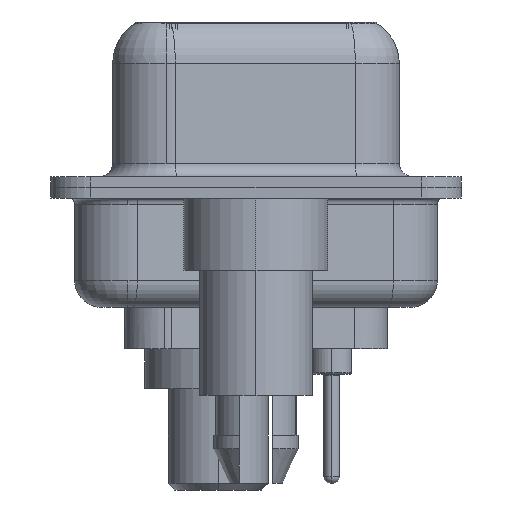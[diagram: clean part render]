
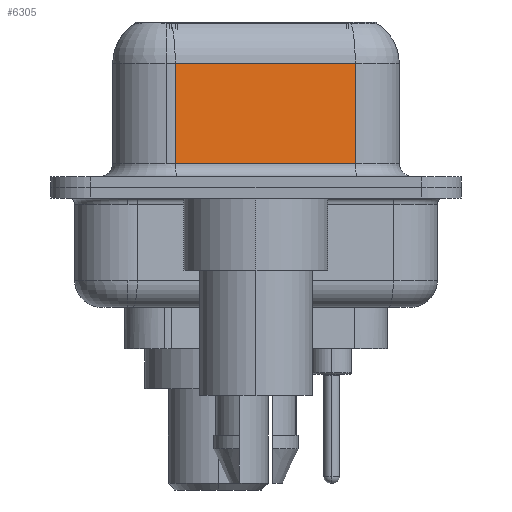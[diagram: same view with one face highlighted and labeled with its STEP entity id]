
A CAD part, left-side view. The second image highlights one B-rep face of the part: STEP entity #6305.
In plain terms, the highlighted planar face has unit normal (-0.985, -0.174, 0).
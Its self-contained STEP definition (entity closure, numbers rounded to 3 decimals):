
#283 = DIRECTION ( 'NONE',  ( -0.174, 0.985, 0. ) ) ;
#1527 = DIRECTION ( 'NONE',  ( 0.985, 0.174, 0. ) ) ;
#2743 = CARTESIAN_POINT ( 'NONE',  ( 5.621, -3.722, 4.65 ) ) ;
#2935 = VECTOR ( 'NONE', #3713, 1000. ) ;
#3349 = ORIENTED_EDGE ( 'NONE', *, *, #15307, .T. ) ;
#3713 = DIRECTION ( 'NONE',  ( 0., 0., -1. ) ) ;
#4613 = LINE ( 'NONE', #24072, #15837 ) ;
#5332 = LINE ( 'NONE', #29730, #9336 ) ;
#5907 = VERTEX_POINT ( 'NONE', #23598 ) ;
#6305 = ADVANCED_FACE ( 'NONE', ( #26242 ), #14415, .F. ) ;
#6557 = ORIENTED_EDGE ( 'NONE', *, *, #26319, .T. ) ;
#7037 = VERTEX_POINT ( 'NONE', #14533 ) ;
#9336 = VECTOR ( 'NONE', #31839, 1000. ) ;
#9765 = CARTESIAN_POINT ( 'NONE',  ( 4.43, 3.028, 0.9 ) ) ;
#11619 = DIRECTION ( 'NONE',  ( -0.174, 0.985, 0. ) ) ;
#13220 = EDGE_CURVE ( 'NONE', #7037, #5907, #26695, .T. ) ;
#13606 = VERTEX_POINT ( 'NONE', #9765 ) ;
#14415 = PLANE ( 'NONE',  #29644 ) ;
#14533 = CARTESIAN_POINT ( 'NONE',  ( 5.621, -3.722, 4.65 ) ) ;
#15307 = EDGE_CURVE ( 'NONE', #13606, #24419, #5332, .T. ) ;
#15837 = VECTOR ( 'NONE', #21283, 1000. ) ;
#16180 = LINE ( 'NONE', #18631, #2935 ) ;
#16942 = EDGE_LOOP ( 'NONE', ( #22038, #29409, #6557, #3349 ) ) ;
#17000 = CARTESIAN_POINT ( 'NONE',  ( 5.621, -3.722, 6.4 ) ) ;
#18631 = CARTESIAN_POINT ( 'NONE',  ( 5.621, -3.722, 6.4 ) ) ;
#19093 = VECTOR ( 'NONE', #283, 1000. ) ;
#21283 = DIRECTION ( 'NONE',  ( 0., 0., -1. ) ) ;
#22038 = ORIENTED_EDGE ( 'NONE', *, *, #27960, .F. ) ;
#22910 = CARTESIAN_POINT ( 'NONE',  ( 5.621, -3.722, 0.9 ) ) ;
#23598 = CARTESIAN_POINT ( 'NONE',  ( 4.43, 3.028, 4.65 ) ) ;
#24072 = CARTESIAN_POINT ( 'NONE',  ( 4.43, 3.028, 6.4 ) ) ;
#24419 = VERTEX_POINT ( 'NONE', #22910 ) ;
#26242 = FACE_OUTER_BOUND ( 'NONE', #16942, .T. ) ;
#26319 = EDGE_CURVE ( 'NONE', #5907, #13606, #4613, .T. ) ;
#26695 = LINE ( 'NONE', #2743, #19093 ) ;
#27960 = EDGE_CURVE ( 'NONE', #7037, #24419, #16180, .T. ) ;
#29409 = ORIENTED_EDGE ( 'NONE', *, *, #13220, .T. ) ;
#29644 = AXIS2_PLACEMENT_3D ( 'NONE', #17000, #1527, #11619 ) ;
#29730 = CARTESIAN_POINT ( 'NONE',  ( 5.621, -3.722, 0.9 ) ) ;
#31839 = DIRECTION ( 'NONE',  ( 0.174, -0.985, 0. ) ) ;
